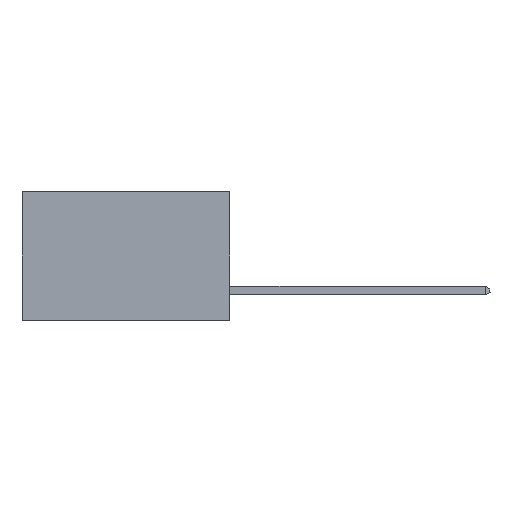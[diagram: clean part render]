
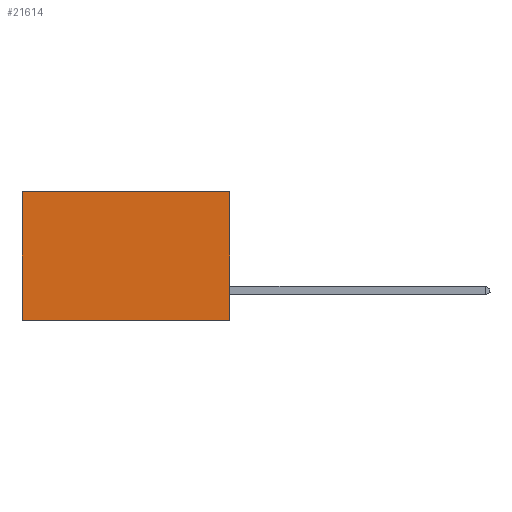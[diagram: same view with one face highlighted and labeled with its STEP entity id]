
A CAD part, left-side view. The second image highlights one B-rep face of the part: STEP entity #21614.
In plain terms, the highlighted planar face has unit normal (-1, 0, 0).
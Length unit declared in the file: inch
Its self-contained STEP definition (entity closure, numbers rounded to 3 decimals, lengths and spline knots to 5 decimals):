
#1862 = EDGE_CURVE ( 'NONE', #7348, #9400, #4288, .T. ) ;
#1907 = PLANE ( 'NONE',  #26098 ) ;
#4288 = LINE ( 'NONE', #13561, #20684 ) ;
#5824 = VECTOR ( 'NONE', #23575, 39.37008 ) ;
#7204 = ORIENTED_EDGE ( 'NONE', *, *, #24114, .F. ) ;
#7348 = VERTEX_POINT ( 'NONE', #17501 ) ;
#8662 = CARTESIAN_POINT ( 'NONE',  ( 0.298, 0., 0. ) ) ;
#8857 = CARTESIAN_POINT ( 'NONE',  ( 0.298, 0., -0.37 ) ) ;
#8871 = ORIENTED_EDGE ( 'NONE', *, *, #1862, .T. ) ;
#9400 = VERTEX_POINT ( 'NONE', #11148 ) ;
#9422 = EDGE_CURVE ( 'NONE', #7348, #24294, #27883, .T. ) ;
#10558 = VECTOR ( 'NONE', #13552, 39.37008 ) ;
#11148 = CARTESIAN_POINT ( 'NONE',  ( 0.298, 0.6, 0. ) ) ;
#11498 = VECTOR ( 'NONE', #17875, 39.37008 ) ;
#11864 = CARTESIAN_POINT ( 'NONE',  ( 0.298, 0., -0.37 ) ) ;
#12128 = VERTEX_POINT ( 'NONE', #25686 ) ;
#13470 = DIRECTION ( 'NONE',  ( 0., 1., 0. ) ) ;
#13552 = DIRECTION ( 'NONE',  ( 0., 1., 0. ) ) ;
#13561 = CARTESIAN_POINT ( 'NONE',  ( 0.298, 0., 0. ) ) ;
#14392 = ORIENTED_EDGE ( 'NONE', *, *, #9422, .F. ) ;
#16156 = EDGE_LOOP ( 'NONE', ( #19876, #7204, #14392, #8871 ) ) ;
#17157 = CARTESIAN_POINT ( 'NONE',  ( 0.298, 0.6, 0. ) ) ;
#17501 = CARTESIAN_POINT ( 'NONE',  ( 0.298, 0., 0. ) ) ;
#17875 = DIRECTION ( 'NONE',  ( 0., 0., -1. ) ) ;
#19876 = ORIENTED_EDGE ( 'NONE', *, *, #21960, .T. ) ;
#19980 = DIRECTION ( 'NONE',  ( 0., 0., -1. ) ) ;
#20105 = CARTESIAN_POINT ( 'NONE',  ( 0.298, 0., 0. ) ) ;
#20684 = VECTOR ( 'NONE', #13470, 39.37008 ) ;
#21614 = ADVANCED_FACE ( 'NONE', ( #24005 ), #1907, .F. ) ;
#21960 = EDGE_CURVE ( 'NONE', #9400, #12128, #23258, .T. ) ;
#23258 = LINE ( 'NONE', #17157, #5824 ) ;
#23575 = DIRECTION ( 'NONE',  ( 0., 0., -1. ) ) ;
#24005 = FACE_OUTER_BOUND ( 'NONE', #16156, .T. ) ;
#24114 = EDGE_CURVE ( 'NONE', #24294, #12128, #25557, .T. ) ;
#24282 = DIRECTION ( 'NONE',  ( 1., 0., 0. ) ) ;
#24294 = VERTEX_POINT ( 'NONE', #11864 ) ;
#25557 = LINE ( 'NONE', #8857, #10558 ) ;
#25686 = CARTESIAN_POINT ( 'NONE',  ( 0.298, 0.6, -0.37 ) ) ;
#26098 = AXIS2_PLACEMENT_3D ( 'NONE', #8662, #24282, #19980 ) ;
#27883 = LINE ( 'NONE', #20105, #11498 ) ;
